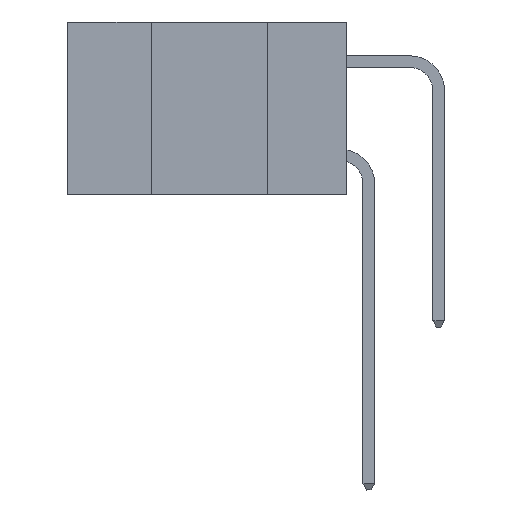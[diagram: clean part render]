
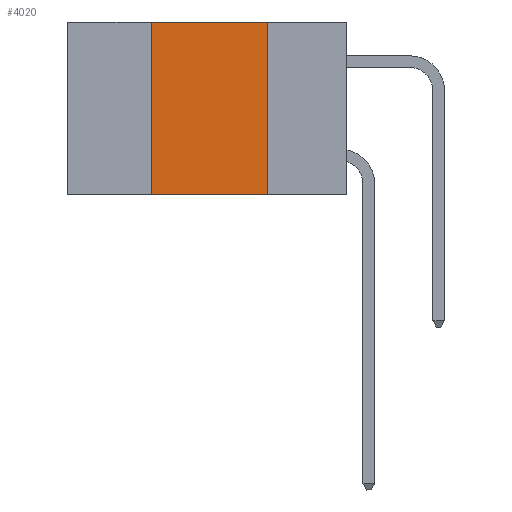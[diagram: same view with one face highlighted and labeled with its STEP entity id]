
A CAD part, left-side view. The second image highlights one B-rep face of the part: STEP entity #4020.
In plain terms, the highlighted planar face has unit normal (-1, 0, 0).
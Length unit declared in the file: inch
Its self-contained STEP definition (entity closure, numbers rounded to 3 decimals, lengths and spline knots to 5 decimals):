
#608 = CARTESIAN_POINT ( 'NONE',  ( 0., 0.6, 0. ) ) ;
#958 = ORIENTED_EDGE ( 'NONE', *, *, #7029, .T. ) ;
#1340 = VECTOR ( 'NONE', #10133, 39.37008 ) ;
#1347 = DIRECTION ( 'NONE',  ( 0., 0., -1. ) ) ;
#1387 = VECTOR ( 'NONE', #13964, 39.37008 ) ;
#1856 = CARTESIAN_POINT ( 'NONE',  ( 0., 0.17, 0. ) ) ;
#2923 = VERTEX_POINT ( 'NONE', #21319 ) ;
#3098 = CARTESIAN_POINT ( 'NONE',  ( 0., 0.42, -0.37 ) ) ;
#4020 = ADVANCED_FACE ( 'NONE', ( #7389 ), #28836, .F. ) ;
#5731 = EDGE_CURVE ( 'NONE', #21876, #2923, #10900, .T. ) ;
#6066 = DIRECTION ( 'NONE',  ( 0., 0., -1. ) ) ;
#7029 = EDGE_CURVE ( 'NONE', #21876, #17332, #7414, .T. ) ;
#7203 = ORIENTED_EDGE ( 'NONE', *, *, #20075, .F. ) ;
#7389 = FACE_OUTER_BOUND ( 'NONE', #13711, .T. ) ;
#7414 = LINE ( 'NONE', #19815, #25923 ) ;
#8110 = AXIS2_PLACEMENT_3D ( 'NONE', #19579, #19389, #6066 ) ;
#10133 = DIRECTION ( 'NONE',  ( 0., 0., 1. ) ) ;
#10900 = LINE ( 'NONE', #15000, #1340 ) ;
#13711 = EDGE_LOOP ( 'NONE', ( #7203, #19466, #18637, #958 ) ) ;
#13964 = DIRECTION ( 'NONE',  ( 0., -1., 0. ) ) ;
#15000 = CARTESIAN_POINT ( 'NONE',  ( 0., 0.42, 0. ) ) ;
#16992 = LINE ( 'NONE', #608, #1387 ) ;
#17332 = VERTEX_POINT ( 'NONE', #25370 ) ;
#18637 = ORIENTED_EDGE ( 'NONE', *, *, #5731, .F. ) ;
#19158 = EDGE_CURVE ( 'NONE', #2923, #25874, #16992, .T. ) ;
#19389 = DIRECTION ( 'NONE',  ( 1., 0., 0. ) ) ;
#19466 = ORIENTED_EDGE ( 'NONE', *, *, #19158, .F. ) ;
#19579 = CARTESIAN_POINT ( 'NONE',  ( 0., 0.6, 0. ) ) ;
#19815 = CARTESIAN_POINT ( 'NONE',  ( 0., 0.6, -0.37 ) ) ;
#20075 = EDGE_CURVE ( 'NONE', #25874, #17332, #24444, .T. ) ;
#20551 = VECTOR ( 'NONE', #1347, 39.37008 ) ;
#21319 = CARTESIAN_POINT ( 'NONE',  ( 0., 0.42, 0. ) ) ;
#21876 = VERTEX_POINT ( 'NONE', #3098 ) ;
#24444 = LINE ( 'NONE', #28361, #20551 ) ;
#25370 = CARTESIAN_POINT ( 'NONE',  ( 0., 0.17, -0.37 ) ) ;
#25874 = VERTEX_POINT ( 'NONE', #1856 ) ;
#25923 = VECTOR ( 'NONE', #26568, 39.37008 ) ;
#26568 = DIRECTION ( 'NONE',  ( 0., -1., 0. ) ) ;
#28361 = CARTESIAN_POINT ( 'NONE',  ( 0., 0.17, 0. ) ) ;
#28836 = PLANE ( 'NONE',  #8110 ) ;
